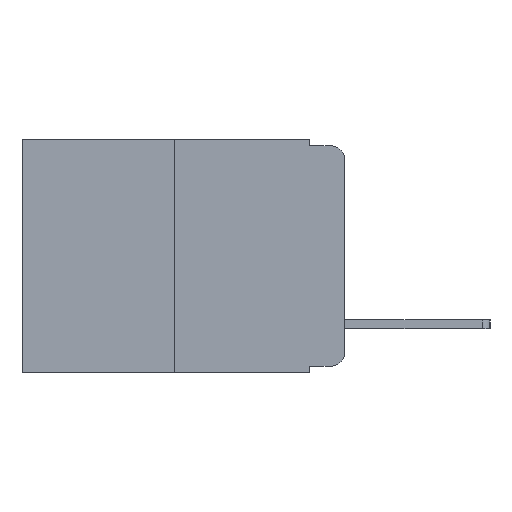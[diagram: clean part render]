
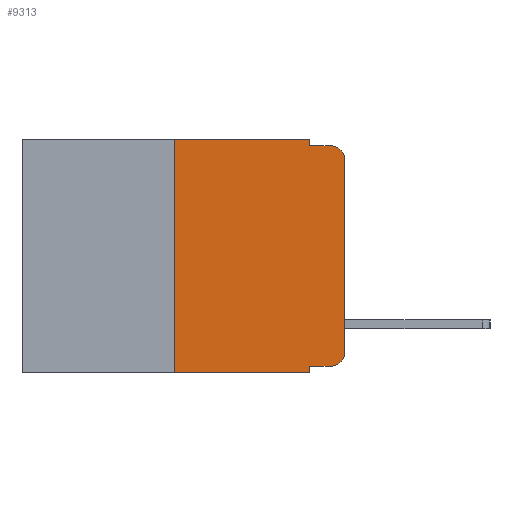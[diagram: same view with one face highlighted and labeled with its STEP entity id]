
A CAD part, left-side view. The second image highlights one B-rep face of the part: STEP entity #9313.
In plain terms, the highlighted planar face has unit normal (-1, 0, 0).
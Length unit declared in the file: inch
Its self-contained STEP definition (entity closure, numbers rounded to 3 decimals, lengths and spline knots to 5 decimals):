
#436 = DIRECTION ( 'NONE',  ( 0., 0., -1. ) ) ;
#476 = ORIENTED_EDGE ( 'NONE', *, *, #13553, .F. ) ;
#534 = VERTEX_POINT ( 'NONE', #3343 ) ;
#1139 = LINE ( 'NONE', #8021, #4792 ) ;
#2206 = ORIENTED_EDGE ( 'NONE', *, *, #17131, .T. ) ;
#2455 = CARTESIAN_POINT ( 'NONE',  ( 0., 0.02, -0.313 ) ) ;
#3171 = LINE ( 'NONE', #16634, #17750 ) ;
#3343 = CARTESIAN_POINT ( 'NONE',  ( 0., 0.25, 0. ) ) ;
#3501 = VERTEX_POINT ( 'NONE', #17201 ) ;
#3928 = CARTESIAN_POINT ( 'NONE',  ( 0., 0., -0.03 ) ) ;
#4036 = DIRECTION ( 'NONE',  ( 0., 0., -1. ) ) ;
#4156 = EDGE_CURVE ( 'NONE', #5227, #5546, #4542, .T. ) ;
#4196 = CARTESIAN_POINT ( 'NONE',  ( 0., 0.02, -0.333 ) ) ;
#4329 = DIRECTION ( 'NONE',  ( 0., 0., -1. ) ) ;
#4542 = LINE ( 'NONE', #4553, #14983 ) ;
#4553 = CARTESIAN_POINT ( 'NONE',  ( 0., 0.473, -0.343 ) ) ;
#4792 = VECTOR ( 'NONE', #12255, 39.37008 ) ;
#5052 = CARTESIAN_POINT ( 'NONE',  ( 0., 0., -0.313 ) ) ;
#5115 = CIRCLE ( 'NONE', #6642, 0.02 ) ;
#5177 = DIRECTION ( 'NONE',  ( 0., 0., -1. ) ) ;
#5227 = VERTEX_POINT ( 'NONE', #17692 ) ;
#5546 = VERTEX_POINT ( 'NONE', #13616 ) ;
#6250 = CARTESIAN_POINT ( 'NONE',  ( 0., 0.25, 0. ) ) ;
#6642 = AXIS2_PLACEMENT_3D ( 'NONE', #17679, #9646, #436 ) ;
#6769 = DIRECTION ( 'NONE',  ( 0., 0., -1. ) ) ;
#7227 = AXIS2_PLACEMENT_3D ( 'NONE', #2455, #12736, #4036 ) ;
#7347 = DIRECTION ( 'NONE',  ( 0., -1., 0. ) ) ;
#7370 = CARTESIAN_POINT ( 'NONE',  ( 0., 0.473, 0. ) ) ;
#7518 = CARTESIAN_POINT ( 'NONE',  ( 0., 0.051, -0.333 ) ) ;
#7571 = LINE ( 'NONE', #8866, #18438 ) ;
#7771 = ORIENTED_EDGE ( 'NONE', *, *, #14433, .F. ) ;
#8021 = CARTESIAN_POINT ( 'NONE',  ( 0., 0., 0. ) ) ;
#8116 = CARTESIAN_POINT ( 'NONE',  ( 0., 0.051, -0.01 ) ) ;
#8173 = CARTESIAN_POINT ( 'NONE',  ( 0., 0.473, 0. ) ) ;
#8247 = ORIENTED_EDGE ( 'NONE', *, *, #4156, .T. ) ;
#8498 = DIRECTION ( 'NONE',  ( 0., -1., 0. ) ) ;
#8866 = CARTESIAN_POINT ( 'NONE',  ( 0., 0.051, 0. ) ) ;
#9184 = ORIENTED_EDGE ( 'NONE', *, *, #12672, .T. ) ;
#9313 = ADVANCED_FACE ( 'NONE', ( #15033 ), #11014, .F. ) ;
#9646 = DIRECTION ( 'NONE',  ( -1., 0., 0. ) ) ;
#9825 = ORIENTED_EDGE ( 'NONE', *, *, #18015, .T. ) ;
#9872 = CARTESIAN_POINT ( 'NONE',  ( 0., 0.02, -0.01 ) ) ;
#10286 = DIRECTION ( 'NONE',  ( 0., -1., 0. ) ) ;
#10673 = ORIENTED_EDGE ( 'NONE', *, *, #16269, .F. ) ;
#10875 = VECTOR ( 'NONE', #6769, 39.37008 ) ;
#11014 = PLANE ( 'NONE',  #17109 ) ;
#11246 = VERTEX_POINT ( 'NONE', #7518 ) ;
#11276 = LINE ( 'NONE', #7370, #17952 ) ;
#11552 = LINE ( 'NONE', #6250, #18609 ) ;
#11771 = EDGE_CURVE ( 'NONE', #12617, #12199, #12370, .T. ) ;
#11958 = VECTOR ( 'NONE', #7347, 39.37008 ) ;
#12199 = VERTEX_POINT ( 'NONE', #5052 ) ;
#12255 = DIRECTION ( 'NONE',  ( 0., 0., 1. ) ) ;
#12370 = CIRCLE ( 'NONE', #7227, 0.02 ) ;
#12372 = LINE ( 'NONE', #12945, #11958 ) ;
#12395 = VERTEX_POINT ( 'NONE', #9872 ) ;
#12617 = VERTEX_POINT ( 'NONE', #4196 ) ;
#12672 = EDGE_CURVE ( 'NONE', #11246, #12617, #12372, .T. ) ;
#12736 = DIRECTION ( 'NONE',  ( -1., 0., 0. ) ) ;
#12945 = CARTESIAN_POINT ( 'NONE',  ( 0., 0.051, -0.333 ) ) ;
#13385 = VERTEX_POINT ( 'NONE', #3928 ) ;
#13553 = EDGE_CURVE ( 'NONE', #11246, #5546, #7571, .T. ) ;
#13616 = CARTESIAN_POINT ( 'NONE',  ( 0., 0.051, -0.343 ) ) ;
#13700 = DIRECTION ( 'NONE',  ( 1., 0., 0. ) ) ;
#13771 = CARTESIAN_POINT ( 'NONE',  ( 0., 0.051, 0. ) ) ;
#14426 = LINE ( 'NONE', #13771, #10875 ) ;
#14433 = EDGE_CURVE ( 'NONE', #5227, #534, #11552, .T. ) ;
#14639 = DIRECTION ( 'NONE',  ( 0., 0., 1. ) ) ;
#14657 = ORIENTED_EDGE ( 'NONE', *, *, #15361, .F. ) ;
#14983 = VECTOR ( 'NONE', #18520, 39.37008 ) ;
#15033 = FACE_OUTER_BOUND ( 'NONE', #17712, .T. ) ;
#15361 = EDGE_CURVE ( 'NONE', #3501, #17100, #14426, .T. ) ;
#16269 = EDGE_CURVE ( 'NONE', #17100, #12395, #3171, .T. ) ;
#16364 = ORIENTED_EDGE ( 'NONE', *, *, #11771, .T. ) ;
#16634 = CARTESIAN_POINT ( 'NONE',  ( 0., 0.051, -0.01 ) ) ;
#17100 = VERTEX_POINT ( 'NONE', #8116 ) ;
#17109 = AXIS2_PLACEMENT_3D ( 'NONE', #8173, #13700, #5177 ) ;
#17131 = EDGE_CURVE ( 'NONE', #13385, #12395, #5115, .T. ) ;
#17201 = CARTESIAN_POINT ( 'NONE',  ( 0., 0.051, 0. ) ) ;
#17591 = EDGE_CURVE ( 'NONE', #534, #3501, #11276, .T. ) ;
#17679 = CARTESIAN_POINT ( 'NONE',  ( 0., 0.02, -0.03 ) ) ;
#17692 = CARTESIAN_POINT ( 'NONE',  ( 0., 0.25, -0.343 ) ) ;
#17712 = EDGE_LOOP ( 'NONE', ( #9825, #2206, #10673, #14657, #18201, #7771, #8247, #476, #9184, #16364 ) ) ;
#17750 = VECTOR ( 'NONE', #8498, 39.37008 ) ;
#17952 = VECTOR ( 'NONE', #10286, 39.37008 ) ;
#18015 = EDGE_CURVE ( 'NONE', #12199, #13385, #1139, .T. ) ;
#18201 = ORIENTED_EDGE ( 'NONE', *, *, #17591, .F. ) ;
#18438 = VECTOR ( 'NONE', #4329, 39.37008 ) ;
#18520 = DIRECTION ( 'NONE',  ( 0., -1., 0. ) ) ;
#18609 = VECTOR ( 'NONE', #14639, 39.37008 ) ;
